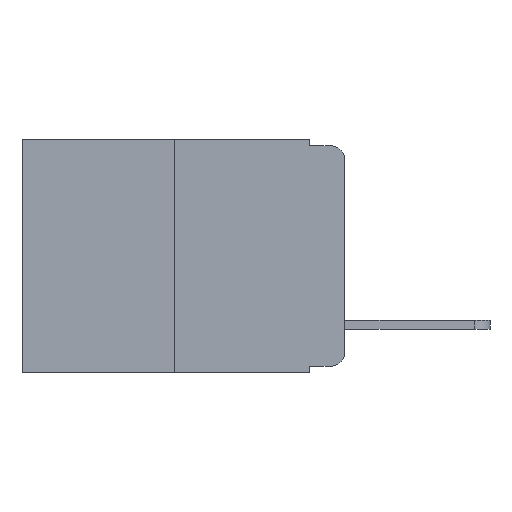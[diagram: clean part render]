
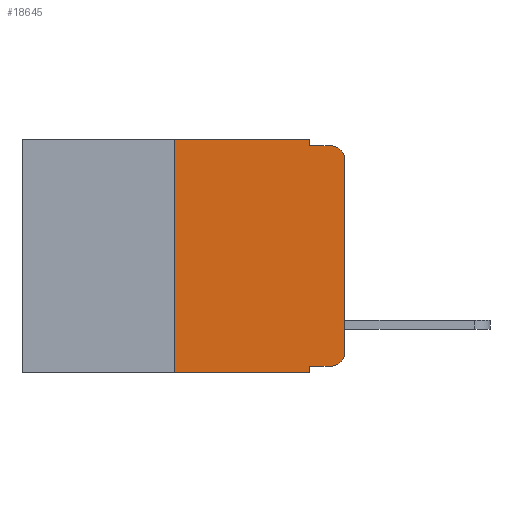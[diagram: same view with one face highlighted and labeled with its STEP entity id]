
A CAD part, left-side view. The second image highlights one B-rep face of the part: STEP entity #18645.
In plain terms, the highlighted planar face has unit normal (-1, 0, 0).
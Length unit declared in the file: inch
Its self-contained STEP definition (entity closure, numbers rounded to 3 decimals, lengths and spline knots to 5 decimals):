
#361 = CARTESIAN_POINT ( 'NONE',  ( 0., 0.051, -0.01 ) ) ;
#817 = CARTESIAN_POINT ( 'NONE',  ( 0., 0.051, 0. ) ) ;
#1880 = PLANE ( 'NONE',  #12412 ) ;
#2322 = LINE ( 'NONE', #7896, #12008 ) ;
#2350 = VERTEX_POINT ( 'NONE', #23164 ) ;
#2404 = CARTESIAN_POINT ( 'NONE',  ( 0., 0.02, -0.313 ) ) ;
#2496 = CARTESIAN_POINT ( 'NONE',  ( 0., 0.051, -0.343 ) ) ;
#2811 = EDGE_CURVE ( 'NONE', #12430, #6283, #13251, .T. ) ;
#3110 = VECTOR ( 'NONE', #19161, 39.37008 ) ;
#4051 = CARTESIAN_POINT ( 'NONE',  ( 0., 0.051, -0.01 ) ) ;
#4422 = DIRECTION ( 'NONE',  ( 0., 0., -1. ) ) ;
#4434 = VECTOR ( 'NONE', #23904, 39.37008 ) ;
#4501 = CARTESIAN_POINT ( 'NONE',  ( 0., 0.051, -0.333 ) ) ;
#4749 = VECTOR ( 'NONE', #9020, 39.37008 ) ;
#5614 = VECTOR ( 'NONE', #18880, 39.37008 ) ;
#5915 = LINE ( 'NONE', #12894, #4749 ) ;
#6011 = VERTEX_POINT ( 'NONE', #15861 ) ;
#6283 = VERTEX_POINT ( 'NONE', #23530 ) ;
#6819 = CIRCLE ( 'NONE', #19797, 0.02 ) ;
#6925 = VERTEX_POINT ( 'NONE', #12849 ) ;
#7344 = VERTEX_POINT ( 'NONE', #2496 ) ;
#7710 = LINE ( 'NONE', #817, #20953 ) ;
#7766 = DIRECTION ( 'NONE',  ( 1., 0., 0. ) ) ;
#7896 = CARTESIAN_POINT ( 'NONE',  ( 0., 0.473, -0.343 ) ) ;
#7942 = CARTESIAN_POINT ( 'NONE',  ( 0., 0., 0. ) ) ;
#9020 = DIRECTION ( 'NONE',  ( 0., 0., 1. ) ) ;
#9251 = CARTESIAN_POINT ( 'NONE',  ( 0., 0.02, -0.01 ) ) ;
#9300 = VERTEX_POINT ( 'NONE', #21334 ) ;
#9637 = VERTEX_POINT ( 'NONE', #361 ) ;
#9865 = DIRECTION ( 'NONE',  ( 0., -1., 0. ) ) ;
#10345 = CARTESIAN_POINT ( 'NONE',  ( 0., 0.25, 0. ) ) ;
#10766 = CIRCLE ( 'NONE', #15466, 0.02 ) ;
#11401 = CARTESIAN_POINT ( 'NONE',  ( 0., 0.473, 0. ) ) ;
#11688 = CARTESIAN_POINT ( 'NONE',  ( 0., 0.051, 0. ) ) ;
#11763 = CARTESIAN_POINT ( 'NONE',  ( 0., 0.02, -0.03 ) ) ;
#12008 = VECTOR ( 'NONE', #9865, 39.37008 ) ;
#12412 = AXIS2_PLACEMENT_3D ( 'NONE', #23623, #7766, #20414 ) ;
#12430 = VERTEX_POINT ( 'NONE', #10345 ) ;
#12849 = CARTESIAN_POINT ( 'NONE',  ( 0., 0.051, -0.333 ) ) ;
#12894 = CARTESIAN_POINT ( 'NONE',  ( 0., 0.25, 0. ) ) ;
#13251 = LINE ( 'NONE', #11401, #3110 ) ;
#13568 = DIRECTION ( 'NONE',  ( 0., 0., -1. ) ) ;
#14453 = LINE ( 'NONE', #7942, #4434 ) ;
#15055 = VECTOR ( 'NONE', #19258, 39.37008 ) ;
#15333 = DIRECTION ( 'NONE',  ( 0., 0., -1. ) ) ;
#15466 = AXIS2_PLACEMENT_3D ( 'NONE', #11763, #23842, #13568 ) ;
#15633 = LINE ( 'NONE', #4501, #15055 ) ;
#15674 = DIRECTION ( 'NONE',  ( -1., 0., 0. ) ) ;
#15784 = EDGE_LOOP ( 'NONE', ( #17418, #17467, #17718, #17738, #17781, #18012, #18153, #18222, #18632, #18773 ) ) ;
#15861 = CARTESIAN_POINT ( 'NONE',  ( 0., 0.25, -0.343 ) ) ;
#16180 = VECTOR ( 'NONE', #15333, 39.37008 ) ;
#16224 = DIRECTION ( 'NONE',  ( 0., 0., -1. ) ) ;
#17418 = ORIENTED_EDGE ( 'NONE', *, *, #20949, .T. ) ;
#17467 = ORIENTED_EDGE ( 'NONE', *, *, #20849, .T. ) ;
#17718 = ORIENTED_EDGE ( 'NONE', *, *, #20847, .F. ) ;
#17738 = ORIENTED_EDGE ( 'NONE', *, *, #20822, .F. ) ;
#17781 = ORIENTED_EDGE ( 'NONE', *, *, #2811, .F. ) ;
#18012 = ORIENTED_EDGE ( 'NONE', *, *, #20352, .F. ) ;
#18153 = ORIENTED_EDGE ( 'NONE', *, *, #22388, .T. ) ;
#18222 = ORIENTED_EDGE ( 'NONE', *, *, #20225, .F. ) ;
#18415 = CARTESIAN_POINT ( 'NONE',  ( 0., 0.02, -0.333 ) ) ;
#18632 = ORIENTED_EDGE ( 'NONE', *, *, #19906, .T. ) ;
#18645 = ADVANCED_FACE ( 'NONE', ( #18715 ), #1880, .F. ) ;
#18715 = FACE_OUTER_BOUND ( 'NONE', #15784, .T. ) ;
#18773 = ORIENTED_EDGE ( 'NONE', *, *, #19794, .T. ) ;
#18880 = DIRECTION ( 'NONE',  ( 0., -1., 0. ) ) ;
#19161 = DIRECTION ( 'NONE',  ( 0., -1., 0. ) ) ;
#19258 = DIRECTION ( 'NONE',  ( 0., -1., 0. ) ) ;
#19267 = VERTEX_POINT ( 'NONE', #9251 ) ;
#19794 = EDGE_CURVE ( 'NONE', #22175, #9300, #6819, .T. ) ;
#19797 = AXIS2_PLACEMENT_3D ( 'NONE', #2404, #15674, #4422 ) ;
#19906 = EDGE_CURVE ( 'NONE', #6925, #22175, #15633, .T. ) ;
#20161 = LINE ( 'NONE', #11688, #16180 ) ;
#20225 = EDGE_CURVE ( 'NONE', #6925, #7344, #7710, .T. ) ;
#20352 = EDGE_CURVE ( 'NONE', #6011, #12430, #5915, .T. ) ;
#20414 = DIRECTION ( 'NONE',  ( 0., 0., -1. ) ) ;
#20686 = LINE ( 'NONE', #4051, #5614 ) ;
#20822 = EDGE_CURVE ( 'NONE', #6283, #9637, #20161, .T. ) ;
#20847 = EDGE_CURVE ( 'NONE', #9637, #19267, #20686, .T. ) ;
#20849 = EDGE_CURVE ( 'NONE', #2350, #19267, #10766, .T. ) ;
#20949 = EDGE_CURVE ( 'NONE', #9300, #2350, #14453, .T. ) ;
#20953 = VECTOR ( 'NONE', #16224, 39.37008 ) ;
#21334 = CARTESIAN_POINT ( 'NONE',  ( 0., 0., -0.313 ) ) ;
#22175 = VERTEX_POINT ( 'NONE', #18415 ) ;
#22388 = EDGE_CURVE ( 'NONE', #6011, #7344, #2322, .T. ) ;
#23164 = CARTESIAN_POINT ( 'NONE',  ( 0., 0., -0.03 ) ) ;
#23530 = CARTESIAN_POINT ( 'NONE',  ( 0., 0.051, 0. ) ) ;
#23623 = CARTESIAN_POINT ( 'NONE',  ( 0., 0.473, 0. ) ) ;
#23842 = DIRECTION ( 'NONE',  ( -1., 0., 0. ) ) ;
#23904 = DIRECTION ( 'NONE',  ( 0., 0., 1. ) ) ;
